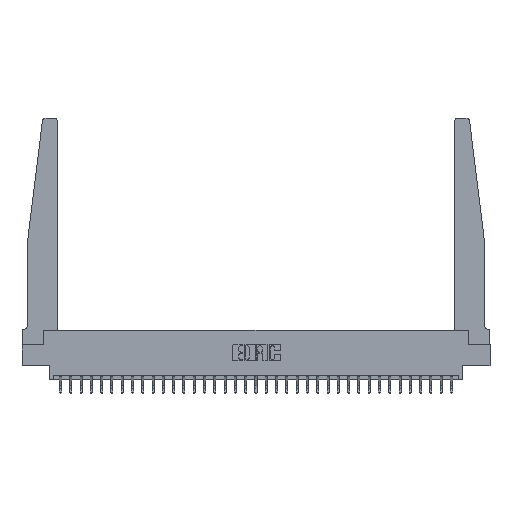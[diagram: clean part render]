
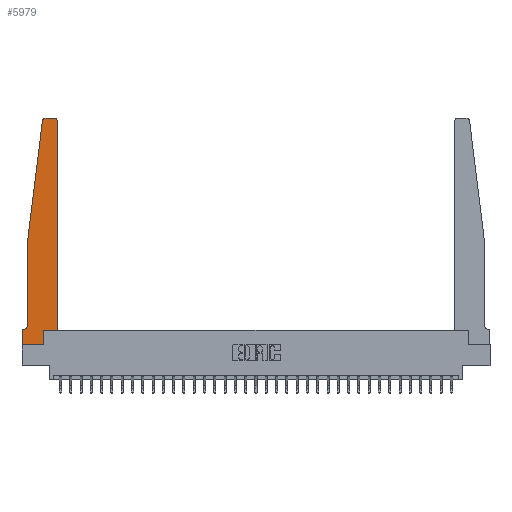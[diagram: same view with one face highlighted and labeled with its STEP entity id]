
A CAD part, top view. The second image highlights one B-rep face of the part: STEP entity #5979.
In plain terms, the highlighted planar face has unit normal (0, 0, 1).
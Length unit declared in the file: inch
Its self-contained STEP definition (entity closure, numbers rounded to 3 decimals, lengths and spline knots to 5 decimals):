
#199 = CARTESIAN_POINT ( 'NONE',  ( 0.425, 2.72, 0.37 ) ) ;
#323 = VERTEX_POINT ( 'NONE', #18715 ) ;
#629 = CARTESIAN_POINT ( 'NONE',  ( 0.425, 0.18, 0.37 ) ) ;
#827 = EDGE_CURVE ( 'NONE', #17973, #323, #22725, .T. ) ;
#1161 = LINE ( 'NONE', #28208, #25104 ) ;
#1476 = EDGE_CURVE ( 'NONE', #21011, #2272, #20501, .T. ) ;
#1743 = EDGE_CURVE ( 'NONE', #5945, #12971, #22370, .T. ) ;
#1784 = EDGE_CURVE ( 'NONE', #24662, #25437, #10433, .T. ) ;
#1977 = DIRECTION ( 'NONE',  ( -1., 0., 0. ) ) ;
#1996 = CIRCLE ( 'NONE', #8082, 0.03 ) ;
#2252 = ORIENTED_EDGE ( 'NONE', *, *, #14405, .T. ) ;
#2272 = VERTEX_POINT ( 'NONE', #12784 ) ;
#2311 = EDGE_CURVE ( 'NONE', #10525, #27185, #22788, .T. ) ;
#2474 = CARTESIAN_POINT ( 'NONE',  ( 0.065, 0.1875, 0.37 ) ) ;
#2695 = CARTESIAN_POINT ( 'NONE',  ( 0.395, 2.75, 0.37 ) ) ;
#2741 = DIRECTION ( 'NONE',  ( 0., 0., 1. ) ) ;
#3124 = DIRECTION ( 'NONE',  ( -0.122, -0.992, 0. ) ) ;
#3289 = CARTESIAN_POINT ( 'NONE',  ( 0.065, 1.25, 0.37 ) ) ;
#3313 = EDGE_CURVE ( 'NONE', #27185, #5945, #3478, .T. ) ;
#3478 = CIRCLE ( 'NONE', #15185, 0.05 ) ;
#3495 = VECTOR ( 'NONE', #15271, 39.37008 ) ;
#3896 = CARTESIAN_POINT ( 'NONE',  ( 0., 0.1875, 0.37 ) ) ;
#4713 = DIRECTION ( 'NONE',  ( -1., 0., 0. ) ) ;
#4920 = VECTOR ( 'NONE', #4713, 39.37008 ) ;
#5297 = CARTESIAN_POINT ( 'NONE',  ( 0., 0.1875, 0.37 ) ) ;
#5506 = CARTESIAN_POINT ( 'NONE',  ( 0.425, 0.18, 0.37 ) ) ;
#5661 = DIRECTION ( 'NONE',  ( 1., 0., 0. ) ) ;
#5945 = VERTEX_POINT ( 'NONE', #22012 ) ;
#5948 = DIRECTION ( 'NONE',  ( 0., -1., 0. ) ) ;
#5979 = ADVANCED_FACE ( 'NONE', ( #10072 ), #24542, .T. ) ;
#7549 = EDGE_LOOP ( 'NONE', ( #29821, #26250, #29154, #27821, #23482, #8058, #16340, #20405, #24415, #29758, #26438, #2252 ) ) ;
#8058 = ORIENTED_EDGE ( 'NONE', *, *, #1743, .T. ) ;
#8082 = AXIS2_PLACEMENT_3D ( 'NONE', #25884, #13189, #23184 ) ;
#8254 = LINE ( 'NONE', #17990, #20956 ) ;
#8348 = DIRECTION ( 'NONE',  ( 0., 1., 0. ) ) ;
#8714 = VECTOR ( 'NONE', #20732, 39.37008 ) ;
#10072 = FACE_OUTER_BOUND ( 'NONE', #7549, .T. ) ;
#10433 = LINE ( 'NONE', #5506, #31309 ) ;
#10525 = VERTEX_POINT ( 'NONE', #18087 ) ;
#10799 = DIRECTION ( 'NONE',  ( 1., 0., 0. ) ) ;
#11206 = CARTESIAN_POINT ( 'NONE',  ( 0.395, 2.72, 0.37 ) ) ;
#12784 = CARTESIAN_POINT ( 'NONE',  ( 0.2605, 0.18, 0.37 ) ) ;
#12971 = VERTEX_POINT ( 'NONE', #3896 ) ;
#13189 = DIRECTION ( 'NONE',  ( 0., 0., 1. ) ) ;
#13256 = CARTESIAN_POINT ( 'NONE',  ( 0.425, 0.18, 0.37 ) ) ;
#14405 = EDGE_CURVE ( 'NONE', #25437, #17973, #21293, .T. ) ;
#15180 = CARTESIAN_POINT ( 'NONE',  ( 0.065, 1.25, 0.37 ) ) ;
#15185 = AXIS2_PLACEMENT_3D ( 'NONE', #18870, #30921, #1977 ) ;
#15242 = EDGE_CURVE ( 'NONE', #323, #24790, #1996, .T. ) ;
#15271 = DIRECTION ( 'NONE',  ( -1., 0., 0. ) ) ;
#15392 = CARTESIAN_POINT ( 'NONE',  ( 0., 0., 0.37 ) ) ;
#16340 = ORIENTED_EDGE ( 'NONE', *, *, #28887, .T. ) ;
#17484 = VECTOR ( 'NONE', #3124, 39.37008 ) ;
#17890 = LINE ( 'NONE', #13256, #8714 ) ;
#17973 = VERTEX_POINT ( 'NONE', #2695 ) ;
#17990 = CARTESIAN_POINT ( 'NONE',  ( 0., 0., 0.37 ) ) ;
#17999 = CARTESIAN_POINT ( 'NONE',  ( 0.24675, 2.72367, 0.37 ) ) ;
#18087 = CARTESIAN_POINT ( 'NONE',  ( 0.065, 1.25, 0.37 ) ) ;
#18141 = EDGE_CURVE ( 'NONE', #27023, #21011, #8254, .T. ) ;
#18715 = CARTESIAN_POINT ( 'NONE',  ( 0.27653, 2.75, 0.37 ) ) ;
#18870 = CARTESIAN_POINT ( 'NONE',  ( 0.015, 0.2375, 0.37 ) ) ;
#19833 = EDGE_CURVE ( 'NONE', #24790, #10525, #24928, .T. ) ;
#20405 = ORIENTED_EDGE ( 'NONE', *, *, #18141, .T. ) ;
#20501 = LINE ( 'NONE', #30173, #25743 ) ;
#20732 = DIRECTION ( 'NONE',  ( 1., 0., 0. ) ) ;
#20763 = AXIS2_PLACEMENT_3D ( 'NONE', #11206, #27441, #5661 ) ;
#20779 = CARTESIAN_POINT ( 'NONE',  ( 0.065, 0.2375, 0.37 ) ) ;
#20956 = VECTOR ( 'NONE', #10799, 39.37008 ) ;
#21011 = VERTEX_POINT ( 'NONE', #21197 ) ;
#21197 = CARTESIAN_POINT ( 'NONE',  ( 0.2605, 0., 0.37 ) ) ;
#21293 = CIRCLE ( 'NONE', #20763, 0.03 ) ;
#22012 = CARTESIAN_POINT ( 'NONE',  ( 0.015, 0.1875, 0.37 ) ) ;
#22370 = LINE ( 'NONE', #2474, #4920 ) ;
#22725 = LINE ( 'NONE', #27008, #3495 ) ;
#22788 = LINE ( 'NONE', #15180, #24775 ) ;
#22838 = AXIS2_PLACEMENT_3D ( 'NONE', #5297, #2741, #24076 ) ;
#23184 = DIRECTION ( 'NONE',  ( 1., 0., 0. ) ) ;
#23482 = ORIENTED_EDGE ( 'NONE', *, *, #3313, .T. ) ;
#24076 = DIRECTION ( 'NONE',  ( 1., 0., 0. ) ) ;
#24415 = ORIENTED_EDGE ( 'NONE', *, *, #1476, .T. ) ;
#24542 = PLANE ( 'NONE',  #22838 ) ;
#24662 = VERTEX_POINT ( 'NONE', #629 ) ;
#24775 = VECTOR ( 'NONE', #29944, 39.37008 ) ;
#24790 = VERTEX_POINT ( 'NONE', #17999 ) ;
#24928 = LINE ( 'NONE', #3289, #17484 ) ;
#25104 = VECTOR ( 'NONE', #5948, 39.37008 ) ;
#25437 = VERTEX_POINT ( 'NONE', #199 ) ;
#25743 = VECTOR ( 'NONE', #27470, 39.37008 ) ;
#25884 = CARTESIAN_POINT ( 'NONE',  ( 0.27653, 2.72, 0.37 ) ) ;
#26236 = EDGE_CURVE ( 'NONE', #2272, #24662, #17890, .T. ) ;
#26250 = ORIENTED_EDGE ( 'NONE', *, *, #15242, .T. ) ;
#26438 = ORIENTED_EDGE ( 'NONE', *, *, #1784, .T. ) ;
#27008 = CARTESIAN_POINT ( 'NONE',  ( 0.25, 2.75, 0.37 ) ) ;
#27023 = VERTEX_POINT ( 'NONE', #15392 ) ;
#27185 = VERTEX_POINT ( 'NONE', #20779 ) ;
#27441 = DIRECTION ( 'NONE',  ( 0., 0., 1. ) ) ;
#27470 = DIRECTION ( 'NONE',  ( 0., 1., 0. ) ) ;
#27821 = ORIENTED_EDGE ( 'NONE', *, *, #2311, .T. ) ;
#28208 = CARTESIAN_POINT ( 'NONE',  ( 0., 0., 0.37 ) ) ;
#28887 = EDGE_CURVE ( 'NONE', #12971, #27023, #1161, .T. ) ;
#29154 = ORIENTED_EDGE ( 'NONE', *, *, #19833, .T. ) ;
#29758 = ORIENTED_EDGE ( 'NONE', *, *, #26236, .T. ) ;
#29821 = ORIENTED_EDGE ( 'NONE', *, *, #827, .T. ) ;
#29944 = DIRECTION ( 'NONE',  ( 0., -1., 0. ) ) ;
#30173 = CARTESIAN_POINT ( 'NONE',  ( 0.2605, 0.18, 0.37 ) ) ;
#30921 = DIRECTION ( 'NONE',  ( 0., 0., -1. ) ) ;
#31309 = VECTOR ( 'NONE', #8348, 39.37008 ) ;
